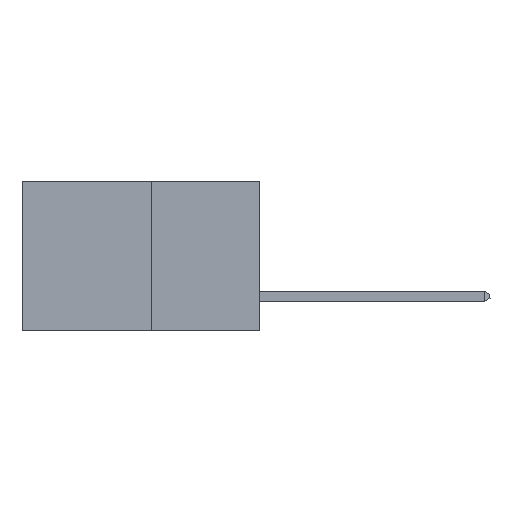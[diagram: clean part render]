
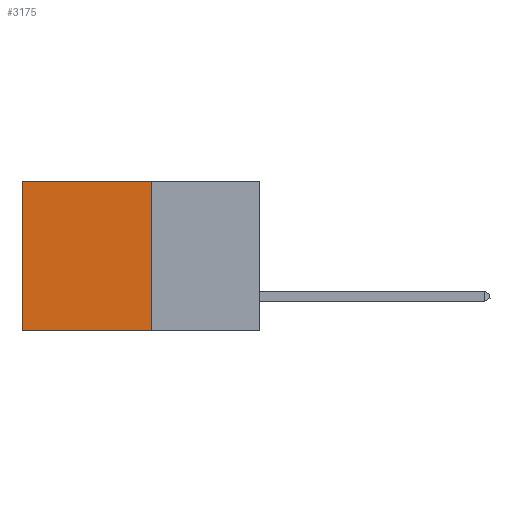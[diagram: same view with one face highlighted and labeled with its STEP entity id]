
A CAD part, left-side view. The second image highlights one B-rep face of the part: STEP entity #3175.
In plain terms, the highlighted planar face has unit normal (-1, 0, 0).
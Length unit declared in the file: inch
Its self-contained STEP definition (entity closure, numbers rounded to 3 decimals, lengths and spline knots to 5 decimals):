
#284 = CARTESIAN_POINT ( 'NONE',  ( 0.277, 0.59, -0.37 ) ) ;
#647 = ORIENTED_EDGE ( 'NONE', *, *, #8753, .F. ) ;
#697 = EDGE_LOOP ( 'NONE', ( #2828, #647, #2812, #2025 ) ) ;
#876 = EDGE_CURVE ( 'NONE', #4457, #5486, #8937, .T. ) ;
#1503 = VERTEX_POINT ( 'NONE', #10673 ) ;
#1799 = CARTESIAN_POINT ( 'NONE',  ( 0.277, 0.27, 0. ) ) ;
#2025 = ORIENTED_EDGE ( 'NONE', *, *, #7006, .T. ) ;
#2086 = EDGE_CURVE ( 'NONE', #1503, #3755, #8632, .T. ) ;
#2361 = DIRECTION ( 'NONE',  ( 0., 0., -1. ) ) ;
#2785 = CARTESIAN_POINT ( 'NONE',  ( 0.277, 0.27, -0.37 ) ) ;
#2812 = ORIENTED_EDGE ( 'NONE', *, *, #876, .F. ) ;
#2828 = ORIENTED_EDGE ( 'NONE', *, *, #2086, .T. ) ;
#2838 = LINE ( 'NONE', #1799, #8111 ) ;
#3175 = ADVANCED_FACE ( 'NONE', ( #4057 ), #11610, .F. ) ;
#3755 = VERTEX_POINT ( 'NONE', #284 ) ;
#3860 = DIRECTION ( 'NONE',  ( 0., 0., -1. ) ) ;
#4057 = FACE_OUTER_BOUND ( 'NONE', #697, .T. ) ;
#4433 = DIRECTION ( 'NONE',  ( 0., 0., -1. ) ) ;
#4457 = VERTEX_POINT ( 'NONE', #5933 ) ;
#4487 = DIRECTION ( 'NONE',  ( 1., 0., 0. ) ) ;
#5486 = VERTEX_POINT ( 'NONE', #11716 ) ;
#5933 = CARTESIAN_POINT ( 'NONE',  ( 0.277, 0.27, 0. ) ) ;
#6019 = CARTESIAN_POINT ( 'NONE',  ( 0.277, 0.59, -0.37 ) ) ;
#6375 = VECTOR ( 'NONE', #2361, 39.37008 ) ;
#6741 = VECTOR ( 'NONE', #11248, 39.37008 ) ;
#7006 = EDGE_CURVE ( 'NONE', #4457, #1503, #2838, .T. ) ;
#8111 = VECTOR ( 'NONE', #8770, 39.37008 ) ;
#8311 = VECTOR ( 'NONE', #3860, 39.37008 ) ;
#8443 = CARTESIAN_POINT ( 'NONE',  ( 0.277, 0.27, -0.37 ) ) ;
#8632 = LINE ( 'NONE', #6019, #8311 ) ;
#8753 = EDGE_CURVE ( 'NONE', #5486, #3755, #9317, .T. ) ;
#8770 = DIRECTION ( 'NONE',  ( 0., 1., 0. ) ) ;
#8937 = LINE ( 'NONE', #2785, #6375 ) ;
#9317 = LINE ( 'NONE', #8443, #6741 ) ;
#9871 = AXIS2_PLACEMENT_3D ( 'NONE', #11967, #4487, #4433 ) ;
#10673 = CARTESIAN_POINT ( 'NONE',  ( 0.277, 0.59, 0. ) ) ;
#11248 = DIRECTION ( 'NONE',  ( 0., 1., 0. ) ) ;
#11610 = PLANE ( 'NONE',  #9871 ) ;
#11716 = CARTESIAN_POINT ( 'NONE',  ( 0.277, 0.27, -0.37 ) ) ;
#11967 = CARTESIAN_POINT ( 'NONE',  ( 0.277, 0.27, -0.37 ) ) ;
